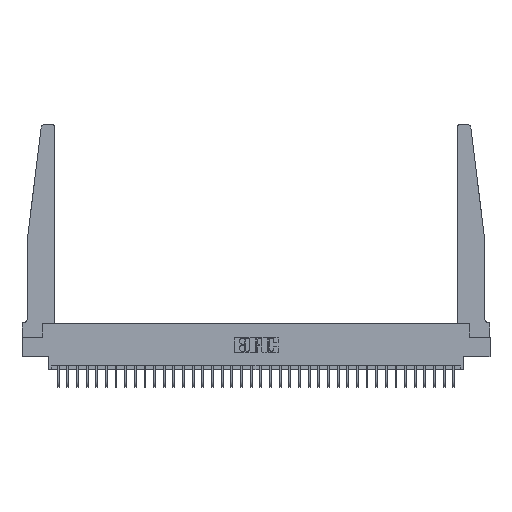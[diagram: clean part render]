
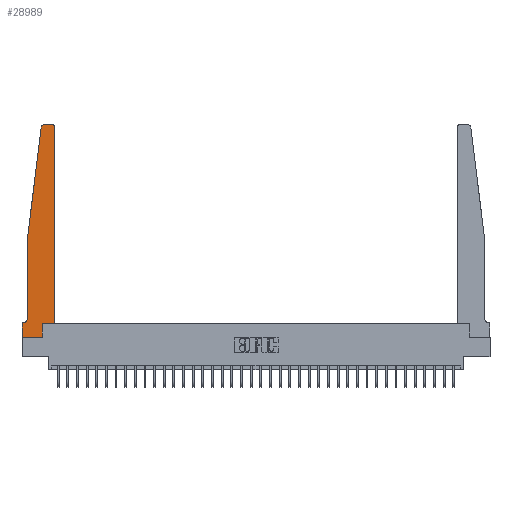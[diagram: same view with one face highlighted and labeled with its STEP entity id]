
A CAD part, top view. The second image highlights one B-rep face of the part: STEP entity #28989.
In plain terms, the highlighted planar face has unit normal (0, 0, 1).
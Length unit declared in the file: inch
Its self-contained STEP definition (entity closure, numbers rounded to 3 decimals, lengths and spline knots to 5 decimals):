
#133 = CARTESIAN_POINT ( 'NONE',  ( 0.2605, 0.18, 0.37 ) ) ;
#693 = VECTOR ( 'NONE', #32962, 39.37008 ) ;
#759 = VECTOR ( 'NONE', #15666, 39.37008 ) ;
#1766 = PLANE ( 'NONE',  #22876 ) ;
#2129 = CARTESIAN_POINT ( 'NONE',  ( 0.425, 0.18, 0.37 ) ) ;
#2424 = EDGE_CURVE ( 'NONE', #28098, #5545, #13963, .T. ) ;
#2871 = EDGE_CURVE ( 'NONE', #2934, #18006, #23715, .T. ) ;
#2934 = VERTEX_POINT ( 'NONE', #10438 ) ;
#3237 = VECTOR ( 'NONE', #16450, 39.37008 ) ;
#4736 = DIRECTION ( 'NONE',  ( 1., 0., 0. ) ) ;
#5385 = VERTEX_POINT ( 'NONE', #34401 ) ;
#5545 = VERTEX_POINT ( 'NONE', #26673 ) ;
#5551 = VERTEX_POINT ( 'NONE', #21242 ) ;
#5577 = VECTOR ( 'NONE', #32909, 39.37008 ) ;
#5767 = EDGE_CURVE ( 'NONE', #9297, #29263, #7085, .T. ) ;
#5879 = CARTESIAN_POINT ( 'NONE',  ( 0., 0., 0.37 ) ) ;
#6362 = AXIS2_PLACEMENT_3D ( 'NONE', #7973, #19113, #29142 ) ;
#6446 = CARTESIAN_POINT ( 'NONE',  ( 0.065, 0.1875, 0.37 ) ) ;
#6563 = EDGE_CURVE ( 'NONE', #5545, #5551, #23403, .T. ) ;
#7018 = FACE_OUTER_BOUND ( 'NONE', #11725, .T. ) ;
#7085 = LINE ( 'NONE', #32969, #17664 ) ;
#7134 = EDGE_CURVE ( 'NONE', #5551, #9297, #30418, .T. ) ;
#7694 = DIRECTION ( 'NONE',  ( 0., 0., 1. ) ) ;
#7707 = AXIS2_PLACEMENT_3D ( 'NONE', #31281, #10440, #23372 ) ;
#7973 = CARTESIAN_POINT ( 'NONE',  ( 0.395, 2.72, 0.37 ) ) ;
#8054 = ORIENTED_EDGE ( 'NONE', *, *, #28405, .T. ) ;
#8351 = AXIS2_PLACEMENT_3D ( 'NONE', #16441, #10702, #16090 ) ;
#8384 = CARTESIAN_POINT ( 'NONE',  ( 0.065, 1.25, 0.37 ) ) ;
#8426 = LINE ( 'NONE', #19057, #3237 ) ;
#8614 = CARTESIAN_POINT ( 'NONE',  ( 0.395, 2.75, 0.37 ) ) ;
#8992 = DIRECTION ( 'NONE',  ( -0.122, -0.992, 0. ) ) ;
#9297 = VERTEX_POINT ( 'NONE', #33015 ) ;
#10293 = ORIENTED_EDGE ( 'NONE', *, *, #25663, .T. ) ;
#10438 = CARTESIAN_POINT ( 'NONE',  ( 0.2605, 0., 0.37 ) ) ;
#10440 = DIRECTION ( 'NONE',  ( 0., 0., 1. ) ) ;
#10702 = DIRECTION ( 'NONE',  ( 0., 0., -1. ) ) ;
#10773 = ORIENTED_EDGE ( 'NONE', *, *, #28882, .T. ) ;
#10844 = DIRECTION ( 'NONE',  ( 0., -1., 0. ) ) ;
#11456 = LINE ( 'NONE', #5879, #693 ) ;
#11725 = EDGE_LOOP ( 'NONE', ( #10773, #10293, #8054, #20541, #15459, #19511, #32176, #33550, #15326, #20205, #26231, #23024 ) ) ;
#11964 = VECTOR ( 'NONE', #17061, 39.37008 ) ;
#13118 = VECTOR ( 'NONE', #10844, 39.37008 ) ;
#13963 = LINE ( 'NONE', #8384, #13118 ) ;
#14171 = LINE ( 'NONE', #24833, #5577 ) ;
#14209 = LINE ( 'NONE', #22416, #16627 ) ;
#15326 = ORIENTED_EDGE ( 'NONE', *, *, #2871, .T. ) ;
#15459 = ORIENTED_EDGE ( 'NONE', *, *, #6563, .T. ) ;
#15666 = DIRECTION ( 'NONE',  ( 0., 1., 0. ) ) ;
#15833 = VERTEX_POINT ( 'NONE', #20805 ) ;
#16090 = DIRECTION ( 'NONE',  ( -1., 0., 0. ) ) ;
#16441 = CARTESIAN_POINT ( 'NONE',  ( 0.015, 0.2375, 0.37 ) ) ;
#16450 = DIRECTION ( 'NONE',  ( 1., 0., 0. ) ) ;
#16627 = VECTOR ( 'NONE', #8992, 39.37008 ) ;
#17061 = DIRECTION ( 'NONE',  ( -1., 0., 0. ) ) ;
#17063 = VECTOR ( 'NONE', #18018, 39.37008 ) ;
#17664 = VECTOR ( 'NONE', #25419, 39.37008 ) ;
#17892 = VERTEX_POINT ( 'NONE', #8614 ) ;
#18006 = VERTEX_POINT ( 'NONE', #24499 ) ;
#18018 = DIRECTION ( 'NONE',  ( 0., 1., 0. ) ) ;
#19040 = VERTEX_POINT ( 'NONE', #25101 ) ;
#19057 = CARTESIAN_POINT ( 'NONE',  ( 0.425, 0.18, 0.37 ) ) ;
#19113 = DIRECTION ( 'NONE',  ( 0., 0., 1. ) ) ;
#19511 = ORIENTED_EDGE ( 'NONE', *, *, #7134, .T. ) ;
#20205 = ORIENTED_EDGE ( 'NONE', *, *, #27420, .T. ) ;
#20541 = ORIENTED_EDGE ( 'NONE', *, *, #2424, .T. ) ;
#20627 = EDGE_CURVE ( 'NONE', #31822, #17892, #31501, .T. ) ;
#20805 = CARTESIAN_POINT ( 'NONE',  ( 0.425, 0.18, 0.37 ) ) ;
#21242 = CARTESIAN_POINT ( 'NONE',  ( 0.015, 0.1875, 0.37 ) ) ;
#21337 = LINE ( 'NONE', #2129, #17063 ) ;
#22416 = CARTESIAN_POINT ( 'NONE',  ( 0.065, 1.25, 0.37 ) ) ;
#22769 = CIRCLE ( 'NONE', #7707, 0.03 ) ;
#22864 = CARTESIAN_POINT ( 'NONE',  ( 0.065, 1.25, 0.37 ) ) ;
#22876 = AXIS2_PLACEMENT_3D ( 'NONE', #28690, #7694, #4736 ) ;
#23024 = ORIENTED_EDGE ( 'NONE', *, *, #20627, .T. ) ;
#23255 = CARTESIAN_POINT ( 'NONE',  ( 0.425, 2.72, 0.37 ) ) ;
#23372 = DIRECTION ( 'NONE',  ( 1., 0., 0. ) ) ;
#23403 = CIRCLE ( 'NONE', #8351, 0.05 ) ;
#23557 = EDGE_CURVE ( 'NONE', #15833, #31822, #21337, .T. ) ;
#23715 = LINE ( 'NONE', #133, #759 ) ;
#24499 = CARTESIAN_POINT ( 'NONE',  ( 0.2605, 0.18, 0.37 ) ) ;
#24833 = CARTESIAN_POINT ( 'NONE',  ( 0.25, 2.75, 0.37 ) ) ;
#25101 = CARTESIAN_POINT ( 'NONE',  ( 0.27653, 2.75, 0.37 ) ) ;
#25419 = DIRECTION ( 'NONE',  ( 0., -1., 0. ) ) ;
#25663 = EDGE_CURVE ( 'NONE', #19040, #5385, #22769, .T. ) ;
#26231 = ORIENTED_EDGE ( 'NONE', *, *, #23557, .T. ) ;
#26673 = CARTESIAN_POINT ( 'NONE',  ( 0.065, 0.2375, 0.37 ) ) ;
#27420 = EDGE_CURVE ( 'NONE', #18006, #15833, #8426, .T. ) ;
#28098 = VERTEX_POINT ( 'NONE', #22864 ) ;
#28405 = EDGE_CURVE ( 'NONE', #5385, #28098, #14209, .T. ) ;
#28690 = CARTESIAN_POINT ( 'NONE',  ( 0., 0.1875, 0.37 ) ) ;
#28882 = EDGE_CURVE ( 'NONE', #17892, #19040, #14171, .T. ) ;
#28989 = ADVANCED_FACE ( 'NONE', ( #7018 ), #1766, .T. ) ;
#29142 = DIRECTION ( 'NONE',  ( 1., 0., 0. ) ) ;
#29263 = VERTEX_POINT ( 'NONE', #33388 ) ;
#30418 = LINE ( 'NONE', #6446, #11964 ) ;
#31281 = CARTESIAN_POINT ( 'NONE',  ( 0.27653, 2.72, 0.37 ) ) ;
#31501 = CIRCLE ( 'NONE', #6362, 0.03 ) ;
#31822 = VERTEX_POINT ( 'NONE', #23255 ) ;
#32176 = ORIENTED_EDGE ( 'NONE', *, *, #5767, .T. ) ;
#32909 = DIRECTION ( 'NONE',  ( -1., 0., 0. ) ) ;
#32962 = DIRECTION ( 'NONE',  ( 1., 0., 0. ) ) ;
#32969 = CARTESIAN_POINT ( 'NONE',  ( 0., 0., 0.37 ) ) ;
#33015 = CARTESIAN_POINT ( 'NONE',  ( 0., 0.1875, 0.37 ) ) ;
#33388 = CARTESIAN_POINT ( 'NONE',  ( 0., 0., 0.37 ) ) ;
#33550 = ORIENTED_EDGE ( 'NONE', *, *, #33942, .T. ) ;
#33942 = EDGE_CURVE ( 'NONE', #29263, #2934, #11456, .T. ) ;
#34401 = CARTESIAN_POINT ( 'NONE',  ( 0.24675, 2.72367, 0.37 ) ) ;
